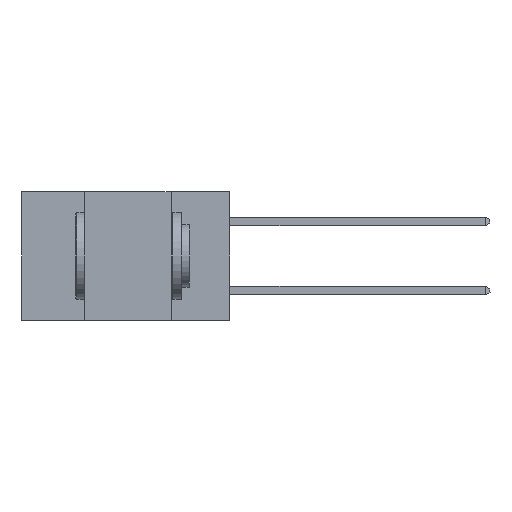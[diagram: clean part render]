
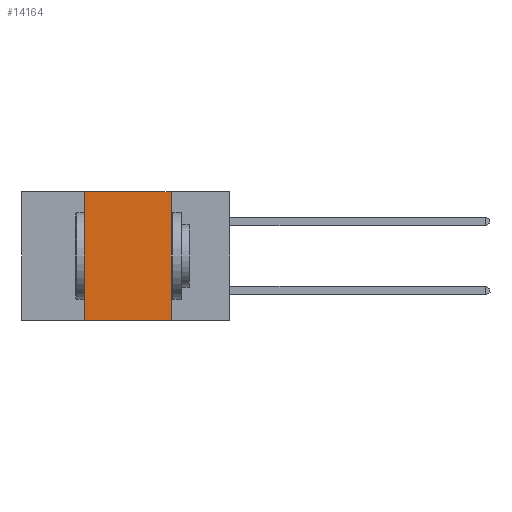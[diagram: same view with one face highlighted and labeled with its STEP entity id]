
A CAD part, left-side view. The second image highlights one B-rep face of the part: STEP entity #14164.
In plain terms, the highlighted planar face has unit normal (-1, 0, 0).
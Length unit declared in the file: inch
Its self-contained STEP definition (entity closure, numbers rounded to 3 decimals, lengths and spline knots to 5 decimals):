
#5 = VERTEX_POINT ( 'NONE', #5717 ) ;
#213 = CARTESIAN_POINT ( 'NONE',  ( 0., 0.17, 0. ) ) ;
#279 = CARTESIAN_POINT ( 'NONE',  ( 0., 0.42, 0. ) ) ;
#1724 = FACE_OUTER_BOUND ( 'NONE', #13301, .T. ) ;
#2119 = LINE ( 'NONE', #7786, #10219 ) ;
#3125 = EDGE_CURVE ( 'NONE', #8886, #8260, #2119, .T. ) ;
#3183 = CARTESIAN_POINT ( 'NONE',  ( 0., 0.17, 0. ) ) ;
#4768 = PLANE ( 'NONE',  #7610 ) ;
#5717 = CARTESIAN_POINT ( 'NONE',  ( 0., 0.17, -0.37 ) ) ;
#6919 = EDGE_CURVE ( 'NONE', #14528, #5, #10368, .T. ) ;
#7610 = AXIS2_PLACEMENT_3D ( 'NONE', #11178, #9999, #13694 ) ;
#7786 = CARTESIAN_POINT ( 'NONE',  ( 0., 0.6, 0. ) ) ;
#7835 = LINE ( 'NONE', #213, #8208 ) ;
#7873 = EDGE_CURVE ( 'NONE', #14528, #8886, #14898, .T. ) ;
#8050 = CARTESIAN_POINT ( 'NONE',  ( 0., 0.6, -0.37 ) ) ;
#8208 = VECTOR ( 'NONE', #15524, 39.37008 ) ;
#8260 = VERTEX_POINT ( 'NONE', #3183 ) ;
#8427 = ORIENTED_EDGE ( 'NONE', *, *, #6919, .T. ) ;
#8886 = VERTEX_POINT ( 'NONE', #12081 ) ;
#9307 = DIRECTION ( 'NONE',  ( 0., -1., 0. ) ) ;
#9999 = DIRECTION ( 'NONE',  ( 1., 0., 0. ) ) ;
#10219 = VECTOR ( 'NONE', #10371, 39.37008 ) ;
#10262 = ORIENTED_EDGE ( 'NONE', *, *, #11956, .F. ) ;
#10368 = LINE ( 'NONE', #8050, #15499 ) ;
#10371 = DIRECTION ( 'NONE',  ( 0., -1., 0. ) ) ;
#11178 = CARTESIAN_POINT ( 'NONE',  ( 0., 0.6, 0. ) ) ;
#11956 = EDGE_CURVE ( 'NONE', #8260, #5, #7835, .T. ) ;
#12081 = CARTESIAN_POINT ( 'NONE',  ( 0., 0.42, 0. ) ) ;
#12395 = ORIENTED_EDGE ( 'NONE', *, *, #7873, .F. ) ;
#12714 = DIRECTION ( 'NONE',  ( 0., 0., 1. ) ) ;
#13301 = EDGE_LOOP ( 'NONE', ( #10262, #14321, #12395, #8427 ) ) ;
#13359 = CARTESIAN_POINT ( 'NONE',  ( 0., 0.42, -0.37 ) ) ;
#13694 = DIRECTION ( 'NONE',  ( 0., 0., -1. ) ) ;
#14164 = ADVANCED_FACE ( 'NONE', ( #1724 ), #4768, .F. ) ;
#14321 = ORIENTED_EDGE ( 'NONE', *, *, #3125, .F. ) ;
#14528 = VERTEX_POINT ( 'NONE', #13359 ) ;
#14898 = LINE ( 'NONE', #279, #15486 ) ;
#15486 = VECTOR ( 'NONE', #12714, 39.37008 ) ;
#15499 = VECTOR ( 'NONE', #9307, 39.37008 ) ;
#15524 = DIRECTION ( 'NONE',  ( 0., 0., -1. ) ) ;
